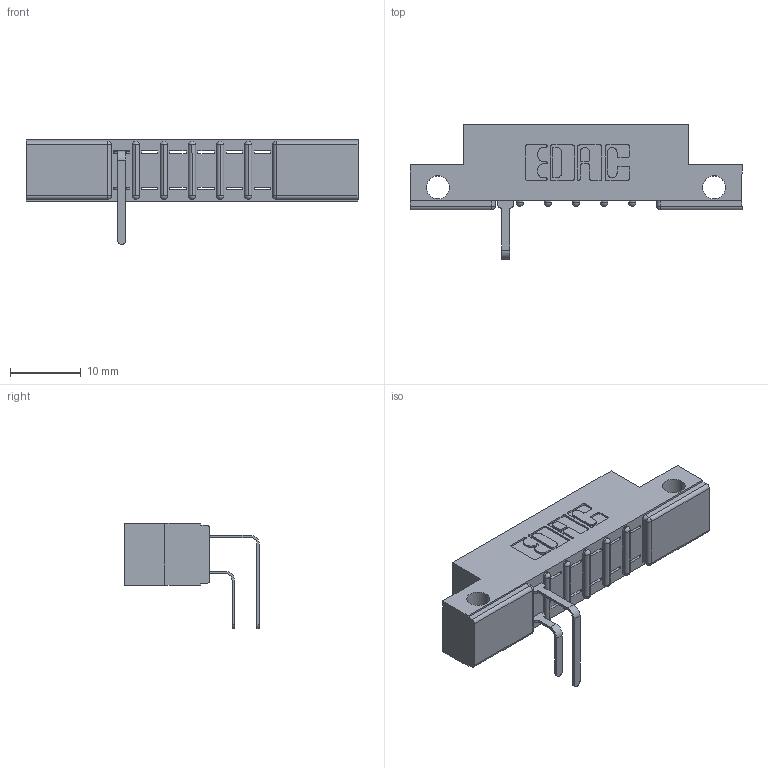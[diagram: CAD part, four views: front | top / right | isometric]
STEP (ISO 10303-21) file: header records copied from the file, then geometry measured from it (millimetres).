
FILE_DESCRIPTION (( 'STEP AP203' ), '1' );
FILE_NAME ('307-006-558-112.STEP', '2018-08-02T18:57:57', ( '' ), ( '' ), 'SwSTEP 2.0', 'SolidWorks 2016', '' );
FILE_SCHEMA (( 'CONFIG_CONTROL_DESIGN' ));
Length unit declared in the file: inch
Products named in the file (4): 307-006-558-112; 307 Part_.128 Dia Side Mounting Holes; 307-290-001_558 559 - 1 (Single); 307-290-001_558 - 2 (Single)
Assembly tree (3 placements, depth 2):
  307-006-558-112
    307 Part_.128 Dia Side Mounting Holes
    307-290-001_558 559 - 1 (Single)
    307-290-001_558 - 2 (Single)
Bounding box: 46.79 x 18.96 x 14.81 mm (x, y, z)
Volume: 2865.6 mm3; surface area: 3374.1 mm2
Topology: 3 solids, 3 shells, 325 faces, 927 edges, 594 vertices
Faces by surface type: plane 196, cylinder 115, sphere 14
Entity records: 10903 total; most frequent: CARTESIAN_POINT 1838, ORIENTED_EDGE 1826, DIRECTION 1805, EDGE_CURVE 913, LINE 683, VECTOR 683, VERTEX_POINT 594, AXIS2_PLACEMENT_3D 561
